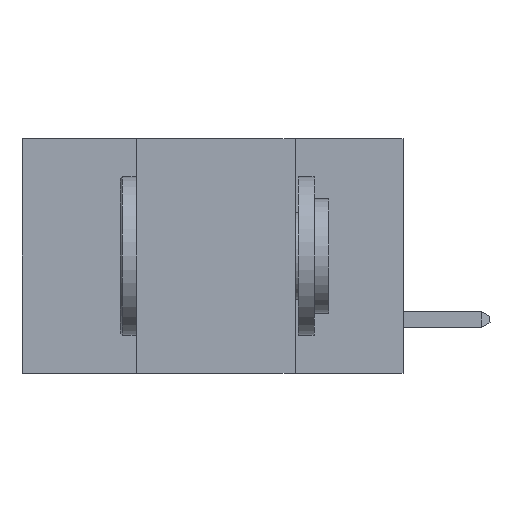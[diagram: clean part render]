
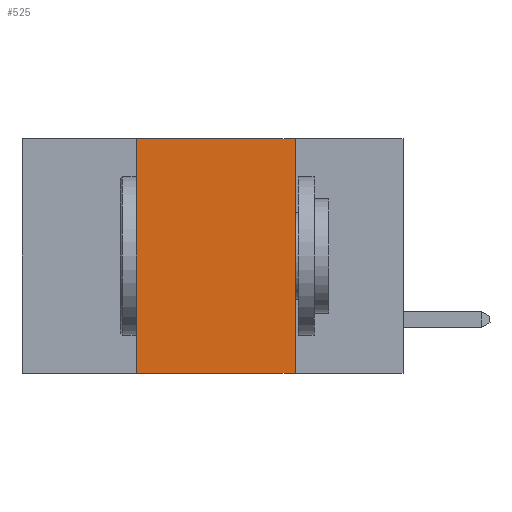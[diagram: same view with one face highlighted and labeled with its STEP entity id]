
A CAD part, left-side view. The second image highlights one B-rep face of the part: STEP entity #525.
In plain terms, the highlighted planar face has unit normal (-1, 0, 0).
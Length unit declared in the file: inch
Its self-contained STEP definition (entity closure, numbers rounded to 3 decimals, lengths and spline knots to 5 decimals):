
#117 = VECTOR ( 'NONE', #2787, 39.37008 ) ;
#135 = LINE ( 'NONE', #9028, #6907 ) ;
#425 = EDGE_LOOP ( 'NONE', ( #9634, #7853, #9860, #3787 ) ) ;
#509 = VERTEX_POINT ( 'NONE', #10598 ) ;
#525 = ADVANCED_FACE ( 'NONE', ( #9693 ), #7950, .F. ) ;
#1800 = DIRECTION ( 'NONE',  ( 0., 0., -1. ) ) ;
#2548 = DIRECTION ( 'NONE',  ( 0., -1., 0. ) ) ;
#2755 = CARTESIAN_POINT ( 'NONE',  ( 0., 0.6, 0. ) ) ;
#2787 = DIRECTION ( 'NONE',  ( 0., -1., 0. ) ) ;
#2831 = CARTESIAN_POINT ( 'NONE',  ( 0., 0.17, -0.37 ) ) ;
#3203 = VERTEX_POINT ( 'NONE', #3519 ) ;
#3206 = CARTESIAN_POINT ( 'NONE',  ( 0., 0.42, 0. ) ) ;
#3342 = VERTEX_POINT ( 'NONE', #2831 ) ;
#3519 = CARTESIAN_POINT ( 'NONE',  ( 0., 0.17, 0. ) ) ;
#3585 = CARTESIAN_POINT ( 'NONE',  ( 0., 0.17, 0. ) ) ;
#3787 = ORIENTED_EDGE ( 'NONE', *, *, #7462, .T. ) ;
#4076 = VECTOR ( 'NONE', #5833, 39.37008 ) ;
#4362 = LINE ( 'NONE', #3206, #4076 ) ;
#4524 = DIRECTION ( 'NONE',  ( 0., 0., -1. ) ) ;
#4608 = AXIS2_PLACEMENT_3D ( 'NONE', #8524, #5607, #1800 ) ;
#5005 = EDGE_CURVE ( 'NONE', #509, #3203, #5300, .T. ) ;
#5300 = LINE ( 'NONE', #2755, #117 ) ;
#5607 = DIRECTION ( 'NONE',  ( 1., 0., 0. ) ) ;
#5833 = DIRECTION ( 'NONE',  ( 0., 0., 1. ) ) ;
#6907 = VECTOR ( 'NONE', #2548, 39.37008 ) ;
#7273 = EDGE_CURVE ( 'NONE', #7422, #509, #4362, .T. ) ;
#7422 = VERTEX_POINT ( 'NONE', #8244 ) ;
#7462 = EDGE_CURVE ( 'NONE', #7422, #3342, #135, .T. ) ;
#7587 = EDGE_CURVE ( 'NONE', #3203, #3342, #7952, .T. ) ;
#7853 = ORIENTED_EDGE ( 'NONE', *, *, #5005, .F. ) ;
#7950 = PLANE ( 'NONE',  #4608 ) ;
#7952 = LINE ( 'NONE', #3585, #9728 ) ;
#8244 = CARTESIAN_POINT ( 'NONE',  ( 0., 0.42, -0.37 ) ) ;
#8524 = CARTESIAN_POINT ( 'NONE',  ( 0., 0.6, 0. ) ) ;
#9028 = CARTESIAN_POINT ( 'NONE',  ( 0., 0.6, -0.37 ) ) ;
#9634 = ORIENTED_EDGE ( 'NONE', *, *, #7587, .F. ) ;
#9693 = FACE_OUTER_BOUND ( 'NONE', #425, .T. ) ;
#9728 = VECTOR ( 'NONE', #4524, 39.37008 ) ;
#9860 = ORIENTED_EDGE ( 'NONE', *, *, #7273, .F. ) ;
#10598 = CARTESIAN_POINT ( 'NONE',  ( 0., 0.42, 0. ) ) ;
